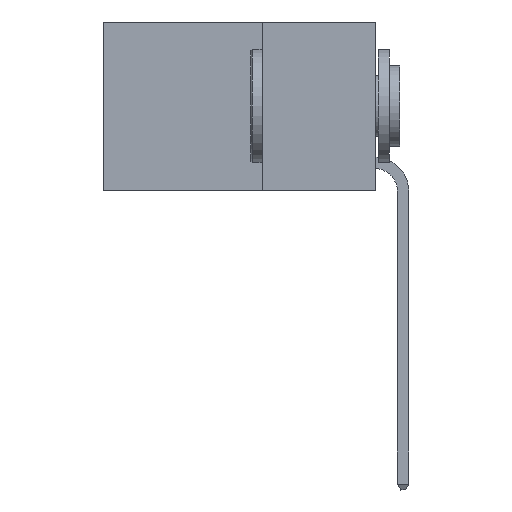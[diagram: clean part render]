
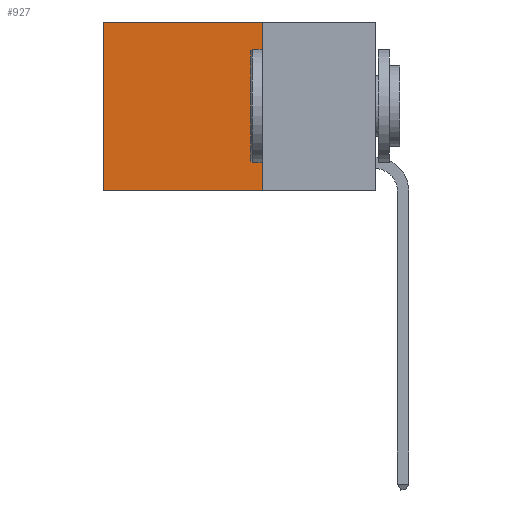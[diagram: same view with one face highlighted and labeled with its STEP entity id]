
A CAD part, left-side view. The second image highlights one B-rep face of the part: STEP entity #927.
In plain terms, the highlighted planar face has unit normal (-1, 0, 0).
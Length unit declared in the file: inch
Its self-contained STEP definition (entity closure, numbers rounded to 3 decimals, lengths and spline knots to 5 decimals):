
#529 = CARTESIAN_POINT ( 'NONE',  ( 0.2625, 0.25, 0. ) ) ;
#927 = ADVANCED_FACE ( 'NONE', ( #6534 ), #8066, .F. ) ;
#1181 = EDGE_CURVE ( 'NONE', #8246, #9100, #7457, .T. ) ;
#1401 = VECTOR ( 'NONE', #7103, 39.37008 ) ;
#1453 = CARTESIAN_POINT ( 'NONE',  ( 0.2625, 0.25, 0. ) ) ;
#1782 = CARTESIAN_POINT ( 'NONE',  ( 0.2625, 0.6, -0.37 ) ) ;
#2602 = VERTEX_POINT ( 'NONE', #15479 ) ;
#2869 = LINE ( 'NONE', #11291, #15637 ) ;
#3675 = CARTESIAN_POINT ( 'NONE',  ( 0.2625, 0.25, -0.37 ) ) ;
#4221 = LINE ( 'NONE', #529, #11141 ) ;
#4446 = EDGE_CURVE ( 'NONE', #2602, #9100, #11230, .T. ) ;
#5330 = DIRECTION ( 'NONE',  ( 1., 0., 0. ) ) ;
#5779 = DIRECTION ( 'NONE',  ( 0., 0., -1. ) ) ;
#6238 = EDGE_LOOP ( 'NONE', ( #8753, #14642, #13081, #7179 ) ) ;
#6534 = FACE_OUTER_BOUND ( 'NONE', #6238, .T. ) ;
#7103 = DIRECTION ( 'NONE',  ( 0., 0., -1. ) ) ;
#7179 = ORIENTED_EDGE ( 'NONE', *, *, #13740, .T. ) ;
#7376 = DIRECTION ( 'NONE',  ( 0., 1., 0. ) ) ;
#7457 = LINE ( 'NONE', #3675, #12928 ) ;
#8066 = PLANE ( 'NONE',  #14583 ) ;
#8246 = VERTEX_POINT ( 'NONE', #8869 ) ;
#8649 = EDGE_CURVE ( 'NONE', #16351, #8246, #4221, .T. ) ;
#8753 = ORIENTED_EDGE ( 'NONE', *, *, #4446, .T. ) ;
#8869 = CARTESIAN_POINT ( 'NONE',  ( 0.2625, 0.25, -0.37 ) ) ;
#9100 = VERTEX_POINT ( 'NONE', #1782 ) ;
#11063 = CARTESIAN_POINT ( 'NONE',  ( 0.2625, 0.6, 0. ) ) ;
#11141 = VECTOR ( 'NONE', #5779, 39.37008 ) ;
#11230 = LINE ( 'NONE', #11063, #1401 ) ;
#11291 = CARTESIAN_POINT ( 'NONE',  ( 0.2625, 0.25, 0. ) ) ;
#12928 = VECTOR ( 'NONE', #7376, 39.37008 ) ;
#13081 = ORIENTED_EDGE ( 'NONE', *, *, #8649, .F. ) ;
#13250 = DIRECTION ( 'NONE',  ( 0., 0., -1. ) ) ;
#13740 = EDGE_CURVE ( 'NONE', #16351, #2602, #2869, .T. ) ;
#14583 = AXIS2_PLACEMENT_3D ( 'NONE', #1453, #5330, #13250 ) ;
#14642 = ORIENTED_EDGE ( 'NONE', *, *, #1181, .F. ) ;
#15162 = DIRECTION ( 'NONE',  ( 0., 1., 0. ) ) ;
#15479 = CARTESIAN_POINT ( 'NONE',  ( 0.2625, 0.6, 0. ) ) ;
#15637 = VECTOR ( 'NONE', #15162, 39.37008 ) ;
#16062 = CARTESIAN_POINT ( 'NONE',  ( 0.2625, 0.25, 0. ) ) ;
#16351 = VERTEX_POINT ( 'NONE', #16062 ) ;
